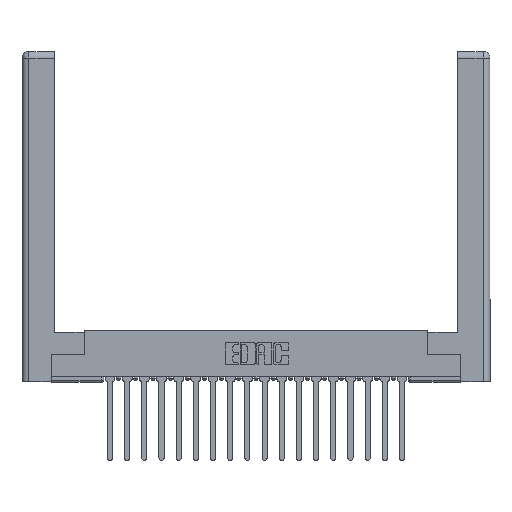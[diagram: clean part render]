
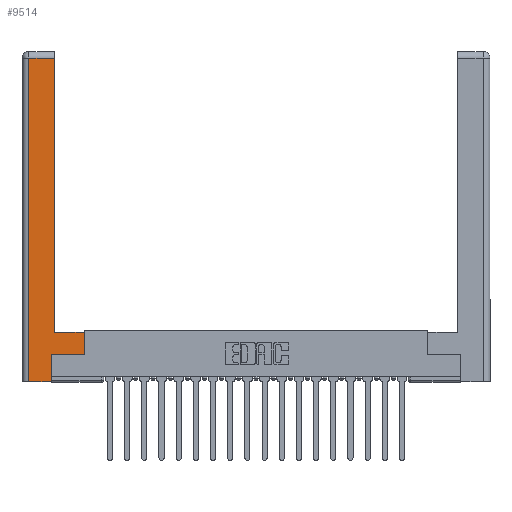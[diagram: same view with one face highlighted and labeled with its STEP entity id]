
A CAD part, top view. The second image highlights one B-rep face of the part: STEP entity #9514.
In plain terms, the highlighted planar face has unit normal (0, 0, 1).
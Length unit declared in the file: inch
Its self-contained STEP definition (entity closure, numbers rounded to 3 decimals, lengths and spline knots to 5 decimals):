
#83 = DIRECTION ( 'NONE',  ( -1., 0., 0. ) ) ;
#182 = VERTEX_POINT ( 'NONE', #20833 ) ;
#420 = CARTESIAN_POINT ( 'NONE',  ( 0.295, 2.94, 0. ) ) ;
#1107 = DIRECTION ( 'NONE',  ( 1., 0., 0. ) ) ;
#1183 = DIRECTION ( 'NONE',  ( -1., 0., 0. ) ) ;
#1192 = VECTOR ( 'NONE', #17649, 39.37008 ) ;
#1290 = CARTESIAN_POINT ( 'NONE',  ( 0.0615, 2.94, 0. ) ) ;
#1341 = LINE ( 'NONE', #12916, #12145 ) ;
#1600 = DIRECTION ( 'NONE',  ( 0., 1., 0. ) ) ;
#1774 = VECTOR ( 'NONE', #7790, 39.37008 ) ;
#1794 = CARTESIAN_POINT ( 'NONE',  ( 0., 0., 0. ) ) ;
#2093 = CARTESIAN_POINT ( 'NONE',  ( 0.0615, 0., 0. ) ) ;
#2283 = VERTEX_POINT ( 'NONE', #6066 ) ;
#2618 = CARTESIAN_POINT ( 'NONE',  ( 0.565, 0.45, 0. ) ) ;
#2682 = LINE ( 'NONE', #1290, #15978 ) ;
#3019 = ORIENTED_EDGE ( 'NONE', *, *, #6306, .T. ) ;
#3032 = EDGE_CURVE ( 'NONE', #7331, #2283, #18890, .T. ) ;
#3120 = ORIENTED_EDGE ( 'NONE', *, *, #7040, .T. ) ;
#3499 = DIRECTION ( 'NONE',  ( 0., 0., -1. ) ) ;
#3507 = ORIENTED_EDGE ( 'NONE', *, *, #18042, .T. ) ;
#4072 = CARTESIAN_POINT ( 'NONE',  ( 0.295, 0.45, 0. ) ) ;
#4864 = DIRECTION ( 'NONE',  ( 0., 1., 0. ) ) ;
#4920 = CARTESIAN_POINT ( 'NONE',  ( 0.565, 0.45, 0. ) ) ;
#5091 = CARTESIAN_POINT ( 'NONE',  ( 0.0615, 2.94, 0. ) ) ;
#5175 = VECTOR ( 'NONE', #1600, 39.37008 ) ;
#5472 = EDGE_LOOP ( 'NONE', ( #3019, #18027, #3507, #10671, #3120, #16212, #16883, #13964 ) ) ;
#6066 = CARTESIAN_POINT ( 'NONE',  ( 0.295, 0.45, 0. ) ) ;
#6076 = DIRECTION ( 'NONE',  ( 0., 1., 0. ) ) ;
#6306 = EDGE_CURVE ( 'NONE', #2283, #10751, #1341, .T. ) ;
#6401 = LINE ( 'NONE', #12647, #12814 ) ;
#6502 = PLANE ( 'NONE',  #15018 ) ;
#7040 = EDGE_CURVE ( 'NONE', #182, #11914, #7654, .T. ) ;
#7331 = VERTEX_POINT ( 'NONE', #2618 ) ;
#7493 = CARTESIAN_POINT ( 'NONE',  ( 0.265, 0.245, 0. ) ) ;
#7654 = LINE ( 'NONE', #7873, #7805 ) ;
#7668 = DIRECTION ( 'NONE',  ( 1., 0., 0. ) ) ;
#7790 = DIRECTION ( 'NONE',  ( -1., 0., 0. ) ) ;
#7805 = VECTOR ( 'NONE', #6076, 39.37008 ) ;
#7873 = CARTESIAN_POINT ( 'NONE',  ( 0.265, 0.245, 0. ) ) ;
#8895 = EDGE_CURVE ( 'NONE', #10751, #11257, #2682, .T. ) ;
#9042 = EDGE_CURVE ( 'NONE', #16250, #7331, #19765, .T. ) ;
#9514 = ADVANCED_FACE ( 'NONE', ( #19734 ), #6502, .F. ) ;
#10105 = LINE ( 'NONE', #14388, #1192 ) ;
#10671 = ORIENTED_EDGE ( 'NONE', *, *, #13264, .T. ) ;
#10751 = VERTEX_POINT ( 'NONE', #420 ) ;
#11257 = VERTEX_POINT ( 'NONE', #5091 ) ;
#11307 = VERTEX_POINT ( 'NONE', #2093 ) ;
#11914 = VERTEX_POINT ( 'NONE', #7493 ) ;
#12145 = VECTOR ( 'NONE', #4864, 39.37008 ) ;
#12274 = CARTESIAN_POINT ( 'NONE',  ( 0.265, 0., 0. ) ) ;
#12479 = LINE ( 'NONE', #12274, #13498 ) ;
#12647 = CARTESIAN_POINT ( 'NONE',  ( 0.565, 0.245, 0. ) ) ;
#12671 = CARTESIAN_POINT ( 'NONE',  ( 0.565, 0.245, 0. ) ) ;
#12814 = VECTOR ( 'NONE', #7668, 39.37008 ) ;
#12916 = CARTESIAN_POINT ( 'NONE',  ( 0.295, 3., 0. ) ) ;
#13264 = EDGE_CURVE ( 'NONE', #11307, #182, #12479, .T. ) ;
#13498 = VECTOR ( 'NONE', #1107, 39.37008 ) ;
#13964 = ORIENTED_EDGE ( 'NONE', *, *, #3032, .T. ) ;
#14388 = CARTESIAN_POINT ( 'NONE',  ( 0.0615, 0., 0. ) ) ;
#15018 = AXIS2_PLACEMENT_3D ( 'NONE', #1794, #3499, #83 ) ;
#15978 = VECTOR ( 'NONE', #1183, 39.37008 ) ;
#16212 = ORIENTED_EDGE ( 'NONE', *, *, #20470, .T. ) ;
#16250 = VERTEX_POINT ( 'NONE', #12671 ) ;
#16883 = ORIENTED_EDGE ( 'NONE', *, *, #9042, .T. ) ;
#17649 = DIRECTION ( 'NONE',  ( 0., -1., 0. ) ) ;
#18027 = ORIENTED_EDGE ( 'NONE', *, *, #8895, .T. ) ;
#18042 = EDGE_CURVE ( 'NONE', #11257, #11307, #10105, .T. ) ;
#18890 = LINE ( 'NONE', #4072, #1774 ) ;
#19734 = FACE_OUTER_BOUND ( 'NONE', #5472, .T. ) ;
#19765 = LINE ( 'NONE', #4920, #5175 ) ;
#20470 = EDGE_CURVE ( 'NONE', #11914, #16250, #6401, .T. ) ;
#20833 = CARTESIAN_POINT ( 'NONE',  ( 0.265, 0., 0. ) ) ;
